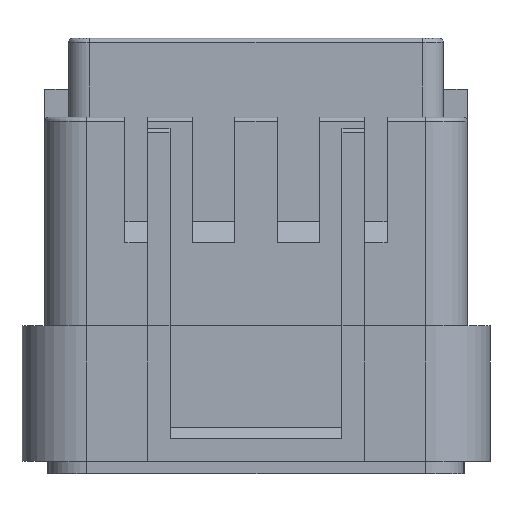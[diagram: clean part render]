
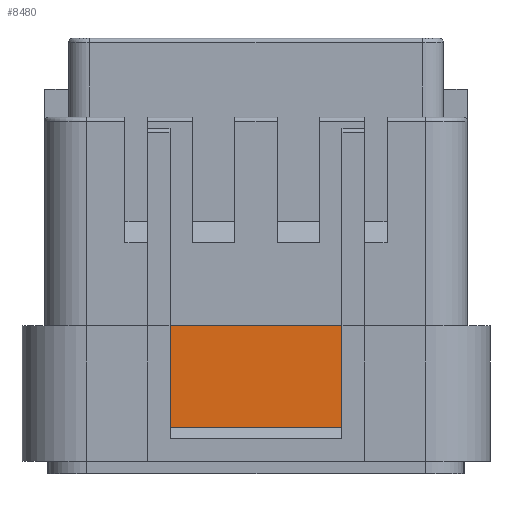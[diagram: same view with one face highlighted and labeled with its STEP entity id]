
A CAD part, front view. The second image highlights one B-rep face of the part: STEP entity #8480.
In plain terms, the highlighted planar face has unit normal (0, -1, 0).
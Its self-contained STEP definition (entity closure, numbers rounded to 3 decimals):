
#55 = CARTESIAN_POINT ( 'NONE',  ( 3.6, -1.55, -14.2 ) ) ;
#315 = PLANE ( 'NONE',  #13602 ) ;
#475 = VECTOR ( 'NONE', #4468, 1000. ) ;
#1440 = VERTEX_POINT ( 'NONE', #7525 ) ;
#1680 = EDGE_CURVE ( 'NONE', #1440, #5147, #8236, .T. ) ;
#2422 = DIRECTION ( 'NONE',  ( 1., 0., 0. ) ) ;
#2696 = VECTOR ( 'NONE', #11939, 1000. ) ;
#3019 = FACE_OUTER_BOUND ( 'NONE', #7634, .T. ) ;
#3099 = CARTESIAN_POINT ( 'NONE',  ( 3.6, -1.55, -10.2 ) ) ;
#3110 = ORIENTED_EDGE ( 'NONE', *, *, #6282, .F. ) ;
#3191 = LINE ( 'NONE', #4642, #2696 ) ;
#3405 = VERTEX_POINT ( 'NONE', #15184 ) ;
#4468 = DIRECTION ( 'NONE',  ( 0., 0., -1. ) ) ;
#4642 = CARTESIAN_POINT ( 'NONE',  ( 12.65, -1.55, -10.2 ) ) ;
#5147 = VERTEX_POINT ( 'NONE', #9753 ) ;
#5221 = CARTESIAN_POINT ( 'NONE',  ( 12.65, -1.55, -15. ) ) ;
#5630 = ORIENTED_EDGE ( 'NONE', *, *, #7423, .T. ) ;
#6282 = EDGE_CURVE ( 'NONE', #3405, #5147, #15594, .T. ) ;
#7205 = VECTOR ( 'NONE', #2422, 1000. ) ;
#7245 = VECTOR ( 'NONE', #13317, 1000. ) ;
#7423 = EDGE_CURVE ( 'NONE', #3405, #14124, #3191, .T. ) ;
#7525 = CARTESIAN_POINT ( 'NONE',  ( 3.6, -1.55, -13.8 ) ) ;
#7634 = EDGE_LOOP ( 'NONE', ( #12372, #12616, #3110, #5630 ) ) ;
#7808 = DIRECTION ( 'NONE',  ( 0., 1., 0. ) ) ;
#8028 = CARTESIAN_POINT ( 'NONE',  ( 9.7, -1.55, -14.2 ) ) ;
#8236 = LINE ( 'NONE', #12057, #7205 ) ;
#8480 = ADVANCED_FACE ( 'NONE', ( #3019 ), #315, .F. ) ;
#9753 = CARTESIAN_POINT ( 'NONE',  ( 9.7, -1.55, -13.8 ) ) ;
#11111 = LINE ( 'NONE', #55, #7245 ) ;
#11939 = DIRECTION ( 'NONE',  ( -1., 0., 0. ) ) ;
#12057 = CARTESIAN_POINT ( 'NONE',  ( 9.7, -1.55, -13.8 ) ) ;
#12372 = ORIENTED_EDGE ( 'NONE', *, *, #14272, .F. ) ;
#12616 = ORIENTED_EDGE ( 'NONE', *, *, #1680, .T. ) ;
#13317 = DIRECTION ( 'NONE',  ( 0., 0., 1. ) ) ;
#13602 = AXIS2_PLACEMENT_3D ( 'NONE', #5221, #7808, #13992 ) ;
#13992 = DIRECTION ( 'NONE',  ( -1., 0., 0. ) ) ;
#14124 = VERTEX_POINT ( 'NONE', #3099 ) ;
#14272 = EDGE_CURVE ( 'NONE', #1440, #14124, #11111, .T. ) ;
#15184 = CARTESIAN_POINT ( 'NONE',  ( 9.7, -1.55, -10.2 ) ) ;
#15594 = LINE ( 'NONE', #8028, #475 ) ;
